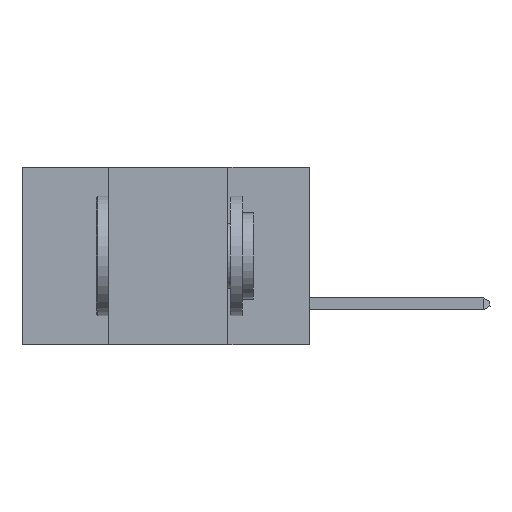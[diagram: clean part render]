
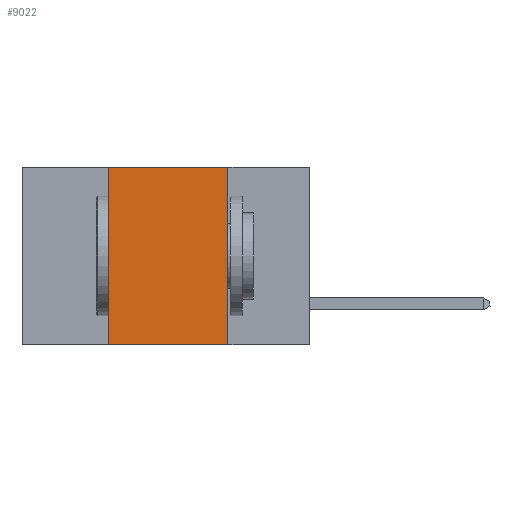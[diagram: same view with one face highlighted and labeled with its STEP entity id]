
A CAD part, left-side view. The second image highlights one B-rep face of the part: STEP entity #9022.
In plain terms, the highlighted planar face has unit normal (-1, 0, 0).
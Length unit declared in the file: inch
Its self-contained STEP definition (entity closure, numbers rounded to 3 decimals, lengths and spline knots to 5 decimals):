
#119 = EDGE_CURVE ( 'NONE', #4162, #5364, #6420, .T. ) ;
#143 = PLANE ( 'NONE',  #1309 ) ;
#182 = DIRECTION ( 'NONE',  ( 0., 0., -1. ) ) ;
#357 = DIRECTION ( 'NONE',  ( 0., -1., 0. ) ) ;
#667 = EDGE_CURVE ( 'NONE', #5364, #8632, #8160, .T. ) ;
#742 = DIRECTION ( 'NONE',  ( 0., -1., 0. ) ) ;
#843 = DIRECTION ( 'NONE',  ( 0., 0., -1. ) ) ;
#1109 = DIRECTION ( 'NONE',  ( 0., 0., 1. ) ) ;
#1228 = EDGE_CURVE ( 'NONE', #8632, #2005, #1826, .T. ) ;
#1309 = AXIS2_PLACEMENT_3D ( 'NONE', #9606, #5290, #182 ) ;
#1735 = CARTESIAN_POINT ( 'NONE',  ( 0., 0.6, 0. ) ) ;
#1826 = LINE ( 'NONE', #5258, #9461 ) ;
#2005 = VERTEX_POINT ( 'NONE', #9887 ) ;
#2086 = ORIENTED_EDGE ( 'NONE', *, *, #1228, .F. ) ;
#2289 = ORIENTED_EDGE ( 'NONE', *, *, #667, .F. ) ;
#2299 = ORIENTED_EDGE ( 'NONE', *, *, #119, .F. ) ;
#2341 = ORIENTED_EDGE ( 'NONE', *, *, #6677, .T. ) ;
#2410 = CARTESIAN_POINT ( 'NONE',  ( 0., 0.42, 0. ) ) ;
#2596 = FACE_OUTER_BOUND ( 'NONE', #4746, .T. ) ;
#4162 = VERTEX_POINT ( 'NONE', #5912 ) ;
#4746 = EDGE_LOOP ( 'NONE', ( #2086, #2289, #2299, #2341 ) ) ;
#5012 = CARTESIAN_POINT ( 'NONE',  ( 0., 0.42, 0. ) ) ;
#5258 = CARTESIAN_POINT ( 'NONE',  ( 0., 0.17, 0. ) ) ;
#5290 = DIRECTION ( 'NONE',  ( 1., 0., 0. ) ) ;
#5364 = VERTEX_POINT ( 'NONE', #2410 ) ;
#5912 = CARTESIAN_POINT ( 'NONE',  ( 0., 0.42, -0.37 ) ) ;
#5982 = VECTOR ( 'NONE', #357, 39.37008 ) ;
#6420 = LINE ( 'NONE', #5012, #8166 ) ;
#6451 = CARTESIAN_POINT ( 'NONE',  ( 0., 0.6, -0.37 ) ) ;
#6677 = EDGE_CURVE ( 'NONE', #4162, #2005, #10146, .T. ) ;
#7047 = VECTOR ( 'NONE', #742, 39.37008 ) ;
#8160 = LINE ( 'NONE', #1735, #5982 ) ;
#8166 = VECTOR ( 'NONE', #1109, 39.37008 ) ;
#8400 = CARTESIAN_POINT ( 'NONE',  ( 0., 0.17, 0. ) ) ;
#8632 = VERTEX_POINT ( 'NONE', #8400 ) ;
#9022 = ADVANCED_FACE ( 'NONE', ( #2596 ), #143, .F. ) ;
#9461 = VECTOR ( 'NONE', #843, 39.37008 ) ;
#9606 = CARTESIAN_POINT ( 'NONE',  ( 0., 0.6, 0. ) ) ;
#9887 = CARTESIAN_POINT ( 'NONE',  ( 0., 0.17, -0.37 ) ) ;
#10146 = LINE ( 'NONE', #6451, #7047 ) ;
